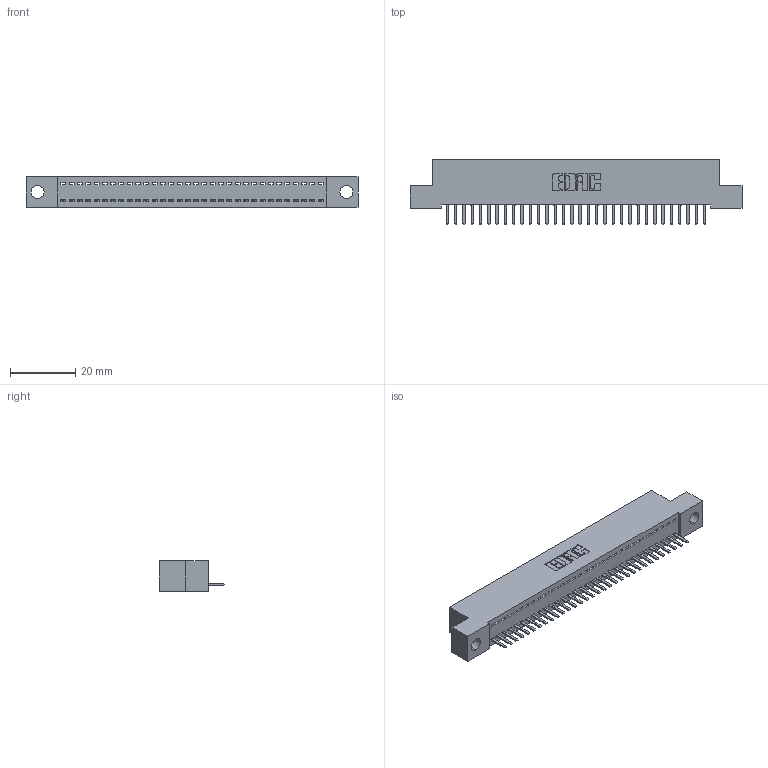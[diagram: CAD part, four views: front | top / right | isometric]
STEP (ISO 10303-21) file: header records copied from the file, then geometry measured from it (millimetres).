
FILE_DESCRIPTION (( 'STEP AP203' ), '1' );
FILE_NAME ('342-032-520-104.STEP', '2018-08-11T16:34:31', ( '' ), ( '' ), 'SwSTEP 2.0', 'SolidWorks 2016', '' );
FILE_SCHEMA (( 'CONFIG_CONTROL_DESIGN' ));
Length unit declared in the file: inch
Products named in the file (3): 342-032-520-104; 342 Part_.156 TH; 345-292-001_345-293-120
Assembly tree (33 placements, depth 2):
  342-032-520-104
    342 Part_.156 TH
    345-292-001_345-293-120  x32
Bounding box: 101.6 x 20.02 x 9.4 mm (x, y, z)
Volume: 8692.4 mm3; surface area: 12102 mm2
Topology: 33 solids, 33 shells, 2094 faces, 6187 edges, 4038 vertices
Faces by surface type: plane 1474, cylinder 620
Entity records: 20841 total; most frequent: CARTESIAN_POINT 3614, ORIENTED_EDGE 3570, DIRECTION 3057, EDGE_CURVE 1785, LINE 1653, VECTOR 1653, VERTEX_POINT 1186, AXIS2_PLACEMENT_3D 702
